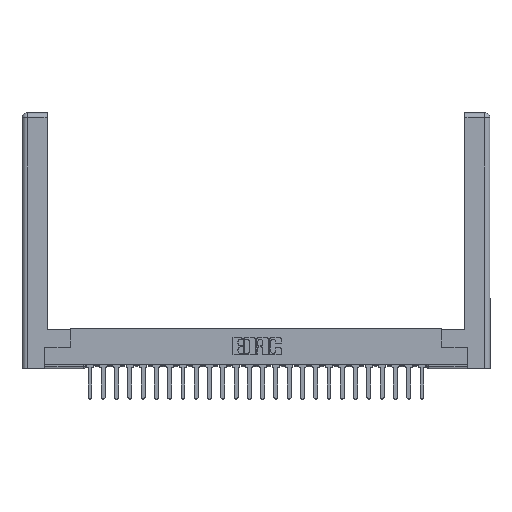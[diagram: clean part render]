
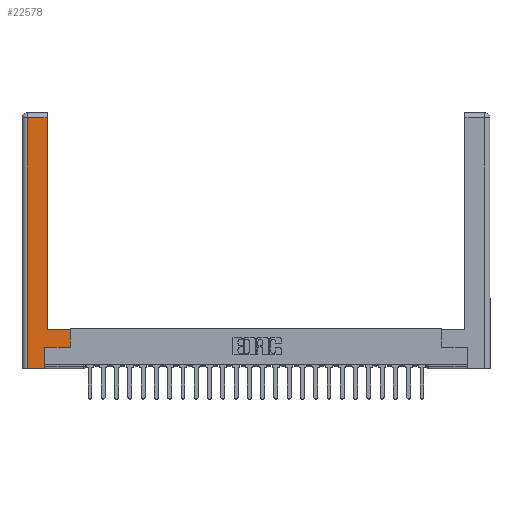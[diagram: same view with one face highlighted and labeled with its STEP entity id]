
A CAD part, top view. The second image highlights one B-rep face of the part: STEP entity #22578.
In plain terms, the highlighted planar face has unit normal (0, 0, 1).
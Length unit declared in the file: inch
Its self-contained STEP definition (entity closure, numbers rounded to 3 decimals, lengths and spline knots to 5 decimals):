
#275 = EDGE_CURVE ( 'NONE', #15098, #3357, #27028, .T. ) ;
#903 = ORIENTED_EDGE ( 'NONE', *, *, #7837, .T. ) ;
#1346 = LINE ( 'NONE', #26816, #22753 ) ;
#1412 = CARTESIAN_POINT ( 'NONE',  ( 0.0615, 2.94, 0. ) ) ;
#2152 = ORIENTED_EDGE ( 'NONE', *, *, #25421, .T. ) ;
#2467 = CARTESIAN_POINT ( 'NONE',  ( 0.0615, 0., 0. ) ) ;
#2683 = ORIENTED_EDGE ( 'NONE', *, *, #7322, .T. ) ;
#2906 = CARTESIAN_POINT ( 'NONE',  ( 0.565, 0.45, 0. ) ) ;
#3200 = ORIENTED_EDGE ( 'NONE', *, *, #26595, .T. ) ;
#3357 = VERTEX_POINT ( 'NONE', #12845 ) ;
#3636 = CARTESIAN_POINT ( 'NONE',  ( 0.265, 0., 0. ) ) ;
#3945 = VECTOR ( 'NONE', #13303, 39.37008 ) ;
#5153 = VERTEX_POINT ( 'NONE', #22303 ) ;
#5248 = DIRECTION ( 'NONE',  ( 0., 0., -1. ) ) ;
#5323 = CARTESIAN_POINT ( 'NONE',  ( 0.565, 0.245, 0. ) ) ;
#6396 = CARTESIAN_POINT ( 'NONE',  ( 0.265, 0.245, 0. ) ) ;
#6629 = EDGE_CURVE ( 'NONE', #17648, #21510, #14848, .T. ) ;
#7070 = LINE ( 'NONE', #22658, #12102 ) ;
#7136 = VECTOR ( 'NONE', #21349, 39.37008 ) ;
#7322 = EDGE_CURVE ( 'NONE', #3357, #14079, #12476, .T. ) ;
#7434 = ORIENTED_EDGE ( 'NONE', *, *, #275, .T. ) ;
#7579 = CARTESIAN_POINT ( 'NONE',  ( 0.565, 0.45, 0. ) ) ;
#7837 = EDGE_CURVE ( 'NONE', #5153, #15098, #7070, .T. ) ;
#8050 = LINE ( 'NONE', #5323, #10727 ) ;
#8551 = EDGE_CURVE ( 'NONE', #21510, #5153, #12737, .T. ) ;
#9237 = CARTESIAN_POINT ( 'NONE',  ( 0.565, 0.245, 0. ) ) ;
#10727 = VECTOR ( 'NONE', #14232, 39.37008 ) ;
#11543 = DIRECTION ( 'NONE',  ( -1., 0., 0. ) ) ;
#12005 = VECTOR ( 'NONE', #16606, 39.37008 ) ;
#12102 = VECTOR ( 'NONE', #18312, 39.37008 ) ;
#12476 = LINE ( 'NONE', #6396, #7136 ) ;
#12737 = LINE ( 'NONE', #1412, #18762 ) ;
#12766 = ORIENTED_EDGE ( 'NONE', *, *, #6629, .T. ) ;
#12845 = CARTESIAN_POINT ( 'NONE',  ( 0.265, 0., 0. ) ) ;
#12874 = VERTEX_POINT ( 'NONE', #7579 ) ;
#13204 = ORIENTED_EDGE ( 'NONE', *, *, #8551, .T. ) ;
#13303 = DIRECTION ( 'NONE',  ( 0., 1., 0. ) ) ;
#14079 = VERTEX_POINT ( 'NONE', #22630 ) ;
#14232 = DIRECTION ( 'NONE',  ( 1., 0., 0. ) ) ;
#14477 = VERTEX_POINT ( 'NONE', #9237 ) ;
#14848 = LINE ( 'NONE', #27292, #16550 ) ;
#15098 = VERTEX_POINT ( 'NONE', #2467 ) ;
#16550 = VECTOR ( 'NONE', #18791, 39.37008 ) ;
#16606 = DIRECTION ( 'NONE',  ( 1., 0., 0. ) ) ;
#16664 = DIRECTION ( 'NONE',  ( -1., 0., 0. ) ) ;
#17648 = VERTEX_POINT ( 'NONE', #22133 ) ;
#18312 = DIRECTION ( 'NONE',  ( 0., -1., 0. ) ) ;
#18430 = ORIENTED_EDGE ( 'NONE', *, *, #25537, .T. ) ;
#18762 = VECTOR ( 'NONE', #20950, 39.37008 ) ;
#18791 = DIRECTION ( 'NONE',  ( 0., 1., 0. ) ) ;
#18956 = CARTESIAN_POINT ( 'NONE',  ( 0., 0., 0. ) ) ;
#19788 = EDGE_LOOP ( 'NONE', ( #12766, #13204, #903, #7434, #2683, #2152, #3200, #18430 ) ) ;
#20950 = DIRECTION ( 'NONE',  ( -1., 0., 0. ) ) ;
#21349 = DIRECTION ( 'NONE',  ( 0., 1., 0. ) ) ;
#21510 = VERTEX_POINT ( 'NONE', #23629 ) ;
#22133 = CARTESIAN_POINT ( 'NONE',  ( 0.295, 0.45, 0. ) ) ;
#22303 = CARTESIAN_POINT ( 'NONE',  ( 0.0615, 2.94, 0. ) ) ;
#22353 = AXIS2_PLACEMENT_3D ( 'NONE', #18956, #5248, #11543 ) ;
#22578 = ADVANCED_FACE ( 'NONE', ( #26448 ), #27707, .F. ) ;
#22630 = CARTESIAN_POINT ( 'NONE',  ( 0.265, 0.245, 0. ) ) ;
#22658 = CARTESIAN_POINT ( 'NONE',  ( 0.0615, 0., 0. ) ) ;
#22753 = VECTOR ( 'NONE', #16664, 39.37008 ) ;
#23629 = CARTESIAN_POINT ( 'NONE',  ( 0.295, 2.94, 0. ) ) ;
#25421 = EDGE_CURVE ( 'NONE', #14079, #14477, #8050, .T. ) ;
#25537 = EDGE_CURVE ( 'NONE', #12874, #17648, #1346, .T. ) ;
#26034 = LINE ( 'NONE', #2906, #3945 ) ;
#26448 = FACE_OUTER_BOUND ( 'NONE', #19788, .T. ) ;
#26595 = EDGE_CURVE ( 'NONE', #14477, #12874, #26034, .T. ) ;
#26816 = CARTESIAN_POINT ( 'NONE',  ( 0.295, 0.45, 0. ) ) ;
#27028 = LINE ( 'NONE', #3636, #12005 ) ;
#27292 = CARTESIAN_POINT ( 'NONE',  ( 0.295, 3., 0. ) ) ;
#27707 = PLANE ( 'NONE',  #22353 ) ;
